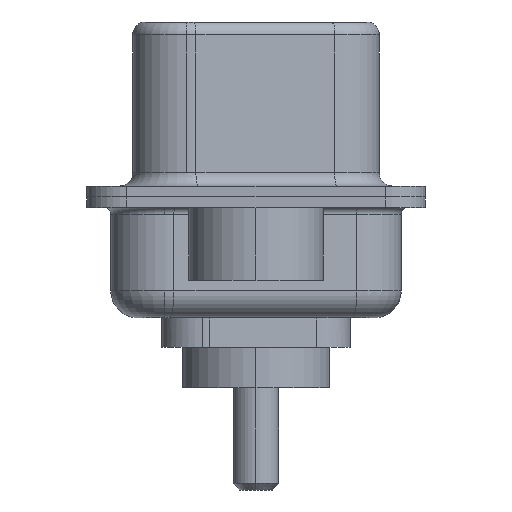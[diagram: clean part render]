
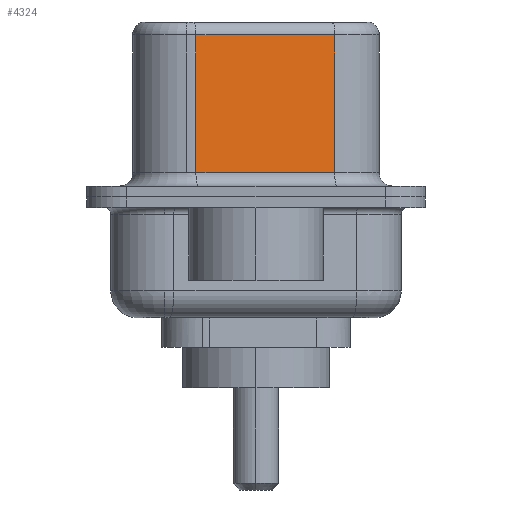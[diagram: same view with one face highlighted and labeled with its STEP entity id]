
A CAD part, left-side view. The second image highlights one B-rep face of the part: STEP entity #4324.
In plain terms, the highlighted planar face has unit normal (-0.985, -0.174, 0).
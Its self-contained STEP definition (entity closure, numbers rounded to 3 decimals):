
#845 = LINE ( 'NONE', #9512, #14094 ) ;
#1524 = DIRECTION ( 'NONE',  ( -0.174, 0.985, 0. ) ) ;
#1535 = ORIENTED_EDGE ( 'NONE', *, *, #9609, .T. ) ;
#1736 = CARTESIAN_POINT ( 'NONE',  ( 4.585, -2.927, 0.9 ) ) ;
#2510 = DIRECTION ( 'NONE',  ( 0.174, -0.985, 0. ) ) ;
#3481 = LINE ( 'NONE', #8852, #6501 ) ;
#3913 = LINE ( 'NONE', #13080, #12382 ) ;
#4137 = VECTOR ( 'NONE', #11967, 1000. ) ;
#4324 = ADVANCED_FACE ( 'NONE', ( #10709 ), #4390, .F. ) ;
#4390 = PLANE ( 'NONE',  #8488 ) ;
#4544 = CARTESIAN_POINT ( 'NONE',  ( 4.585, -2.927, 6.52 ) ) ;
#5000 = EDGE_CURVE ( 'NONE', #6436, #12529, #7652, .T. ) ;
#5011 = DIRECTION ( 'NONE',  ( -0.174, 0.985, 0. ) ) ;
#5085 = CARTESIAN_POINT ( 'NONE',  ( 3.675, 2.233, 6.02 ) ) ;
#5913 = VERTEX_POINT ( 'NONE', #16493 ) ;
#6436 = VERTEX_POINT ( 'NONE', #10873 ) ;
#6501 = VECTOR ( 'NONE', #8451, 1000. ) ;
#7652 = LINE ( 'NONE', #4544, #4137 ) ;
#8451 = DIRECTION ( 'NONE',  ( 0., 0., -1. ) ) ;
#8488 = AXIS2_PLACEMENT_3D ( 'NONE', #9792, #16138, #5011 ) ;
#8852 = CARTESIAN_POINT ( 'NONE',  ( 3.675, 2.233, 6.52 ) ) ;
#8933 = ORIENTED_EDGE ( 'NONE', *, *, #15594, .T. ) ;
#9043 = ORIENTED_EDGE ( 'NONE', *, *, #5000, .F. ) ;
#9450 = ORIENTED_EDGE ( 'NONE', *, *, #14399, .T. ) ;
#9512 = CARTESIAN_POINT ( 'NONE',  ( 4.585, -2.927, 6.02 ) ) ;
#9609 = EDGE_CURVE ( 'NONE', #13134, #5913, #3481, .T. ) ;
#9792 = CARTESIAN_POINT ( 'NONE',  ( 4.585, -2.927, 6.52 ) ) ;
#10709 = FACE_OUTER_BOUND ( 'NONE', #12160, .T. ) ;
#10873 = CARTESIAN_POINT ( 'NONE',  ( 4.585, -2.927, 6.02 ) ) ;
#11967 = DIRECTION ( 'NONE',  ( 0., 0., -1. ) ) ;
#12160 = EDGE_LOOP ( 'NONE', ( #9043, #9450, #1535, #8933 ) ) ;
#12382 = VECTOR ( 'NONE', #2510, 1000. ) ;
#12529 = VERTEX_POINT ( 'NONE', #1736 ) ;
#13080 = CARTESIAN_POINT ( 'NONE',  ( 4.585, -2.927, 0.9 ) ) ;
#13134 = VERTEX_POINT ( 'NONE', #5085 ) ;
#14094 = VECTOR ( 'NONE', #1524, 1000. ) ;
#14399 = EDGE_CURVE ( 'NONE', #6436, #13134, #845, .T. ) ;
#15594 = EDGE_CURVE ( 'NONE', #5913, #12529, #3913, .T. ) ;
#16138 = DIRECTION ( 'NONE',  ( 0.985, 0.174, 0. ) ) ;
#16493 = CARTESIAN_POINT ( 'NONE',  ( 3.675, 2.233, 0.9 ) ) ;
